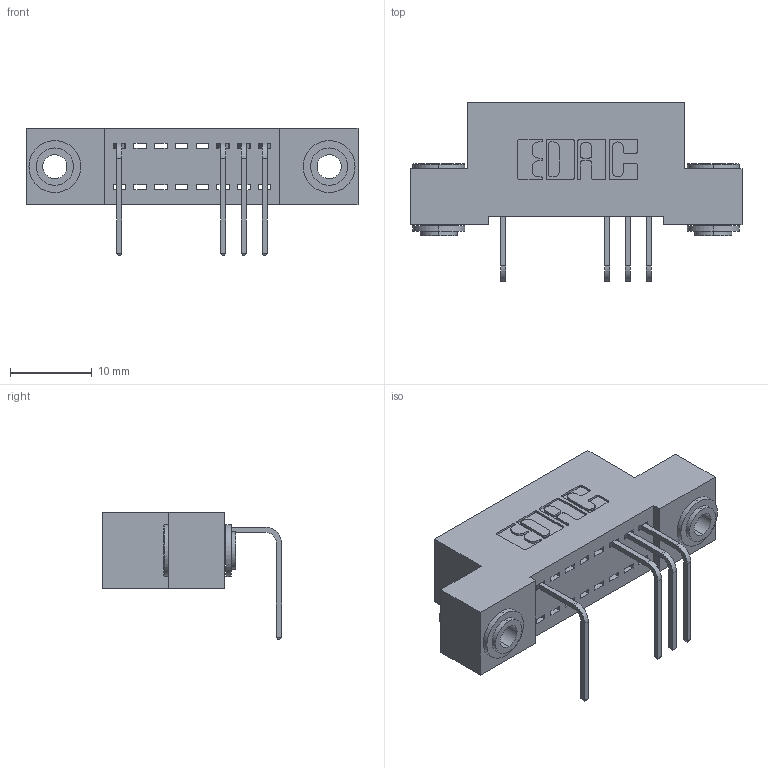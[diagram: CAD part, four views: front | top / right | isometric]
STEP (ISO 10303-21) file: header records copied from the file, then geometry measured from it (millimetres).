
FILE_DESCRIPTION (( 'STEP AP203' ), '1' );
FILE_NAME ('342-008-558-103.STEP', '2018-08-10T12:33:15', ( '' ), ( '' ), 'SwSTEP 2.0', 'SolidWorks 2016', '' );
FILE_SCHEMA (( 'CONFIG_CONTROL_DESIGN' ));
Length unit declared in the file: inch
Products named in the file (4): 342 Part_.156 TH; 345-292-001_558 Tail - 2; 342-250-002_345-250-002-102; 342-008-558-103
Assembly tree (7 placements, depth 2):
  342-008-558-103
    342 Part_.156 TH
    345-292-001_558 Tail - 2  x4
    342-250-002_345-250-002-102  x2
Bounding box: 40.64 x 21.91 x 15.62 mm (x, y, z)
Volume: 3428.5 mm3; surface area: 4464.5 mm2
Topology: 7 solids, 7 shells, 436 faces, 1271 edges, 838 vertices
Faces by surface type: plane 300, cylinder 128, cone 8
Entity records: 9762 total; most frequent: CARTESIAN_POINT 1685, ORIENTED_EDGE 1626, DIRECTION 1519, EDGE_CURVE 813, LINE 661, VECTOR 661, VERTEX_POINT 538, AXIS2_PLACEMENT_3D 429
